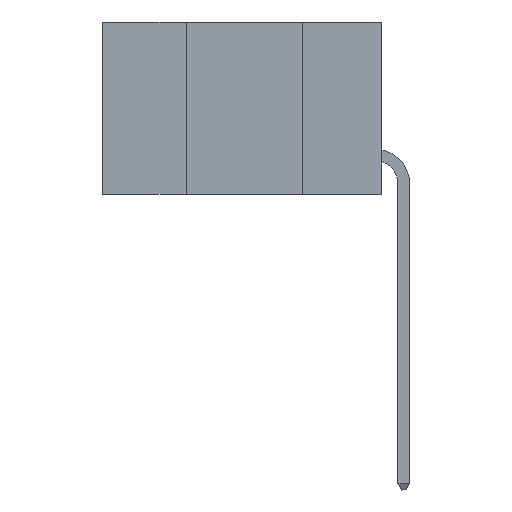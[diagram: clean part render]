
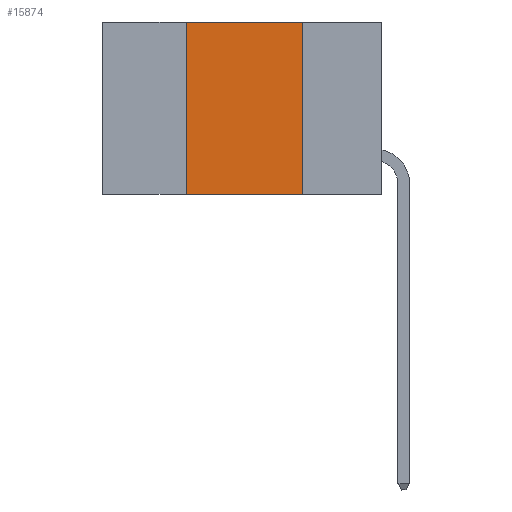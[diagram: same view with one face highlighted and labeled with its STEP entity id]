
A CAD part, left-side view. The second image highlights one B-rep face of the part: STEP entity #15874.
In plain terms, the highlighted planar face has unit normal (-1, 0, 0).
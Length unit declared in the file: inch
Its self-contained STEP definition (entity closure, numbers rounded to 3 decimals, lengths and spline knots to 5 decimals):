
#482 = CARTESIAN_POINT ( 'NONE',  ( 0., 0.42, 0. ) ) ;
#765 = DIRECTION ( 'NONE',  ( 0., -1., 0. ) ) ;
#1223 = CARTESIAN_POINT ( 'NONE',  ( 0., 0.17, 0. ) ) ;
#1418 = FACE_OUTER_BOUND ( 'NONE', #15762, .T. ) ;
#1478 = VERTEX_POINT ( 'NONE', #3382 ) ;
#3382 = CARTESIAN_POINT ( 'NONE',  ( 0., 0.17, -0.37 ) ) ;
#3656 = PLANE ( 'NONE',  #18105 ) ;
#4518 = VECTOR ( 'NONE', #7203, 39.37008 ) ;
#4626 = LINE ( 'NONE', #482, #10092 ) ;
#5546 = CARTESIAN_POINT ( 'NONE',  ( 0., 0.42, 0. ) ) ;
#5633 = VECTOR ( 'NONE', #765, 39.37008 ) ;
#5747 = DIRECTION ( 'NONE',  ( 0., -1., 0. ) ) ;
#6351 = VERTEX_POINT ( 'NONE', #15752 ) ;
#6381 = DIRECTION ( 'NONE',  ( 0., 0., -1. ) ) ;
#7203 = DIRECTION ( 'NONE',  ( 0., 0., -1. ) ) ;
#7716 = ORIENTED_EDGE ( 'NONE', *, *, #8658, .T. ) ;
#8054 = CARTESIAN_POINT ( 'NONE',  ( 0., 0.17, 0. ) ) ;
#8536 = VECTOR ( 'NONE', #5747, 39.37008 ) ;
#8658 = EDGE_CURVE ( 'NONE', #6351, #1478, #10291, .T. ) ;
#9150 = CARTESIAN_POINT ( 'NONE',  ( 0., 0.6, 0. ) ) ;
#10092 = VECTOR ( 'NONE', #13515, 39.37008 ) ;
#10291 = LINE ( 'NONE', #11295, #8536 ) ;
#10536 = ORIENTED_EDGE ( 'NONE', *, *, #17863, .F. ) ;
#10717 = EDGE_CURVE ( 'NONE', #13380, #13230, #16372, .T. ) ;
#11295 = CARTESIAN_POINT ( 'NONE',  ( 0., 0.6, -0.37 ) ) ;
#12806 = ORIENTED_EDGE ( 'NONE', *, *, #10717, .F. ) ;
#12849 = LINE ( 'NONE', #1223, #4518 ) ;
#13230 = VERTEX_POINT ( 'NONE', #8054 ) ;
#13380 = VERTEX_POINT ( 'NONE', #5546 ) ;
#13515 = DIRECTION ( 'NONE',  ( 0., 0., 1. ) ) ;
#14660 = EDGE_CURVE ( 'NONE', #13230, #1478, #12849, .T. ) ;
#15752 = CARTESIAN_POINT ( 'NONE',  ( 0., 0.42, -0.37 ) ) ;
#15762 = EDGE_LOOP ( 'NONE', ( #16617, #12806, #10536, #7716 ) ) ;
#15874 = ADVANCED_FACE ( 'NONE', ( #1418 ), #3656, .F. ) ;
#16075 = CARTESIAN_POINT ( 'NONE',  ( 0., 0.6, 0. ) ) ;
#16136 = DIRECTION ( 'NONE',  ( 1., 0., 0. ) ) ;
#16372 = LINE ( 'NONE', #9150, #5633 ) ;
#16617 = ORIENTED_EDGE ( 'NONE', *, *, #14660, .F. ) ;
#17863 = EDGE_CURVE ( 'NONE', #6351, #13380, #4626, .T. ) ;
#18105 = AXIS2_PLACEMENT_3D ( 'NONE', #16075, #16136, #6381 ) ;
